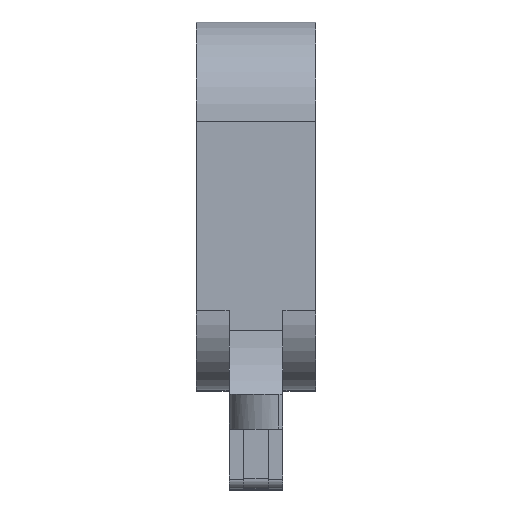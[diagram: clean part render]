
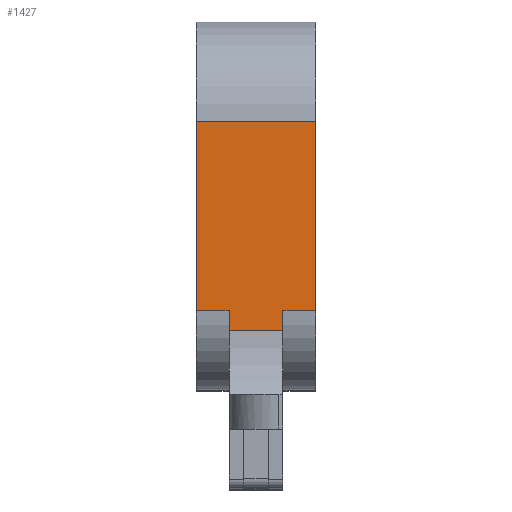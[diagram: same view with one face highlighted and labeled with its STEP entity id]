
A CAD part, top view. The second image highlights one B-rep face of the part: STEP entity #1427.
In plain terms, the highlighted planar face has unit normal (0, 0, 1).
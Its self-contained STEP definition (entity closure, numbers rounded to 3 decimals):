
#535=CARTESIAN_POINT('',(-2.7,-10.0,-66.0));
#536=VERTEX_POINT('',#535);
#544=CARTESIAN_POINT('',(-2.7,-8.,-66.0));
#545=VERTEX_POINT('',#544);
#546=CARTESIAN_POINT('',(-2.7,-8.,-66.0));
#547=DIRECTION('',(0.0,-1.0,0.0));
#548=VECTOR('',#547,2.);
#549=LINE('',#546,#548);
#550=EDGE_CURVE('',#545,#536,#549,.T.);
#870=CARTESIAN_POINT('',(6.,11.,-66.0));
#871=VERTEX_POINT('',#870);
#879=CARTESIAN_POINT('',(6.,-8.,-66.0));
#880=VERTEX_POINT('',#879);
#881=CARTESIAN_POINT('',(6.,-8.,-66.0));
#882=DIRECTION('',(0.0,1.0,0.0));
#883=VECTOR('',#882,19.);
#884=LINE('',#881,#883);
#885=EDGE_CURVE('',#880,#871,#884,.T.);
#1003=CARTESIAN_POINT('',(-6.,-8.,-66.0));
#1004=VERTEX_POINT('',#1003);
#1012=CARTESIAN_POINT('',(-6.,11.,-66.0));
#1013=VERTEX_POINT('',#1012);
#1014=CARTESIAN_POINT('',(-6.,11.,-66.0));
#1015=DIRECTION('',(0.0,-1.0,0.0));
#1016=VECTOR('',#1015,19.);
#1017=LINE('',#1014,#1016);
#1018=EDGE_CURVE('',#1013,#1004,#1017,.T.);
#1322=CARTESIAN_POINT('',(2.7,-10.0,-66.0));
#1323=VERTEX_POINT('',#1322);
#1331=CARTESIAN_POINT('',(2.7,-10.0,-66.0));
#1332=DIRECTION('',(-1.0,0.0,0.0));
#1333=VECTOR('',#1332,5.4);
#1334=LINE('',#1331,#1333);
#1335=EDGE_CURVE('',#1323,#536,#1334,.T.);
#1386=CARTESIAN_POINT('',(-2.7,-8.,-66.0));
#1387=DIRECTION('',(-1.0,0.0,0.0));
#1388=VECTOR('',#1387,3.3);
#1389=LINE('',#1386,#1388);
#1390=EDGE_CURVE('',#545,#1004,#1389,.T.);
#1395=CARTESIAN_POINT('',(0.0,-20.0,-66.0));
#1396=DIRECTION('',(0.0,0.0,1.0));
#1397=DIRECTION('',(1.0,0.0,0.0));
#1398=AXIS2_PLACEMENT_3D('',#1395,#1396,#1397);
#1399=PLANE('',#1398);
#1400=ORIENTED_EDGE('',*,*,#1335,.F.);
#1401=CARTESIAN_POINT('',(2.7,-8.,-66.0));
#1402=VERTEX_POINT('',#1401);
#1403=CARTESIAN_POINT('',(2.7,-8.,-66.0));
#1404=DIRECTION('',(0.0,-1.0,0.0));
#1405=VECTOR('',#1404,2.);
#1406=LINE('',#1403,#1405);
#1407=EDGE_CURVE('',#1402,#1323,#1406,.T.);
#1408=ORIENTED_EDGE('',*,*,#1407,.F.);
#1409=CARTESIAN_POINT('',(6.,-8.,-66.0));
#1410=DIRECTION('',(-1.0,0.0,0.0));
#1411=VECTOR('',#1410,3.3);
#1412=LINE('',#1409,#1411);
#1413=EDGE_CURVE('',#880,#1402,#1412,.T.);
#1414=ORIENTED_EDGE('',*,*,#1413,.F.);
#1415=ORIENTED_EDGE('',*,*,#885,.T.);
#1416=CARTESIAN_POINT('',(-6.,11.,-66.0));
#1417=DIRECTION('',(1.0,0.0,0.0));
#1418=VECTOR('',#1417,12.);
#1419=LINE('',#1416,#1418);
#1420=EDGE_CURVE('',#1013,#871,#1419,.T.);
#1421=ORIENTED_EDGE('',*,*,#1420,.F.);
#1422=ORIENTED_EDGE('',*,*,#1018,.T.);
#1423=ORIENTED_EDGE('',*,*,#1390,.F.);
#1424=ORIENTED_EDGE('',*,*,#550,.T.);
#1425=EDGE_LOOP('',(#1400,#1408,#1414,#1415,#1421,#1422,#1423,#1424));
#1426=FACE_OUTER_BOUND('',#1425,.T.);
#1427=ADVANCED_FACE('',(#1426),#1399,.T.);
